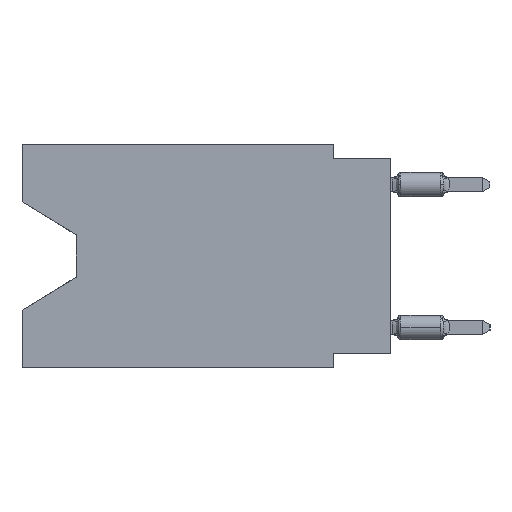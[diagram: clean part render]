
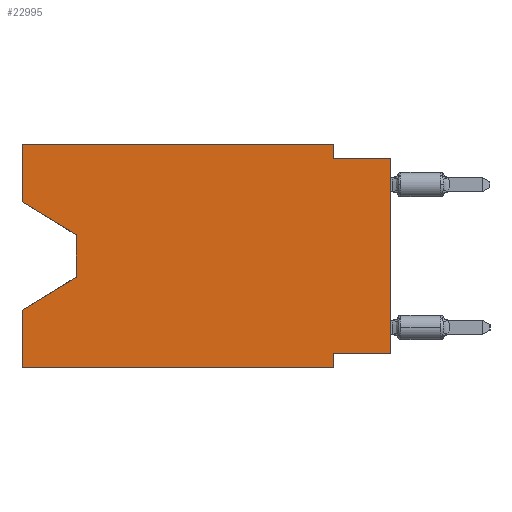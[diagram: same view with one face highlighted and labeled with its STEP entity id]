
A CAD part, left-side view. The second image highlights one B-rep face of the part: STEP entity #22995.
In plain terms, the highlighted planar face has unit normal (-1, 0, 0).
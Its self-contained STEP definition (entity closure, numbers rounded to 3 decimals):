
#367 = CARTESIAN_POINT ( 'NONE',  ( 0., 2.54, -9.906 ) ) ;
#491 = EDGE_LOOP ( 'NONE', ( #17704, #5832, #23189, #4879, #27209, #18446, #586, #12905, #18353, #7124, #14202, #2330 ) ) ;
#516 = VERTEX_POINT ( 'NONE', #23426 ) ;
#586 = ORIENTED_EDGE ( 'NONE', *, *, #18438, .F. ) ;
#728 = EDGE_CURVE ( 'NONE', #2733, #9744, #24272, .T. ) ;
#1650 = LINE ( 'NONE', #8018, #10307 ) ;
#2138 = VERTEX_POINT ( 'NONE', #7632 ) ;
#2330 = ORIENTED_EDGE ( 'NONE', *, *, #15231, .F. ) ;
#2733 = VERTEX_POINT ( 'NONE', #7737 ) ;
#2897 = DIRECTION ( 'NONE',  ( 0., 0., 1. ) ) ;
#3535 = VECTOR ( 'NONE', #8153, 1000. ) ;
#3934 = EDGE_CURVE ( 'NONE', #516, #22753, #12090, .T. ) ;
#4527 = LINE ( 'NONE', #24346, #5271 ) ;
#4879 = ORIENTED_EDGE ( 'NONE', *, *, #18583, .F. ) ;
#5035 = PLANE ( 'NONE',  #27947 ) ;
#5097 = CARTESIAN_POINT ( 'NONE',  ( 0., 16.383, -7.36 ) ) ;
#5271 = VECTOR ( 'NONE', #19856, 1000. ) ;
#5822 = CARTESIAN_POINT ( 'NONE',  ( 0., 16.383, -2.546 ) ) ;
#5832 = ORIENTED_EDGE ( 'NONE', *, *, #3934, .T. ) ;
#6000 = CARTESIAN_POINT ( 'NONE',  ( 0., 13.97, -4.013 ) ) ;
#6475 = CARTESIAN_POINT ( 'NONE',  ( 0., 13.97, -5.893 ) ) ;
#7124 = ORIENTED_EDGE ( 'NONE', *, *, #23572, .F. ) ;
#7632 = CARTESIAN_POINT ( 'NONE',  ( 0., 2.54, -9.271 ) ) ;
#7737 = CARTESIAN_POINT ( 'NONE',  ( 0., 2.54, -0.635 ) ) ;
#8018 = CARTESIAN_POINT ( 'NONE',  ( 0., 16.383, -2.546 ) ) ;
#8153 = DIRECTION ( 'NONE',  ( 0., 0., 1. ) ) ;
#8291 = EDGE_CURVE ( 'NONE', #10574, #18259, #15759, .T. ) ;
#8428 = LINE ( 'NONE', #24194, #14132 ) ;
#8631 = CARTESIAN_POINT ( 'NONE',  ( 0., 16.383, 0. ) ) ;
#9358 = EDGE_CURVE ( 'NONE', #19790, #28056, #4527, .T. ) ;
#9383 = DIRECTION ( 'NONE',  ( 0., -1., 0. ) ) ;
#9526 = VERTEX_POINT ( 'NONE', #12427 ) ;
#9607 = EDGE_CURVE ( 'NONE', #22753, #18701, #10807, .T. ) ;
#9618 = CARTESIAN_POINT ( 'NONE',  ( 0., 0., -9.271 ) ) ;
#9744 = VERTEX_POINT ( 'NONE', #24423 ) ;
#10307 = VECTOR ( 'NONE', #16832, 1000. ) ;
#10445 = VECTOR ( 'NONE', #25067, 1000. ) ;
#10574 = VERTEX_POINT ( 'NONE', #11309 ) ;
#10807 = LINE ( 'NONE', #6475, #17264 ) ;
#11309 = CARTESIAN_POINT ( 'NONE',  ( 0., 16.383, -9.906 ) ) ;
#11474 = VECTOR ( 'NONE', #13114, 1000. ) ;
#11920 = VECTOR ( 'NONE', #12233, 1000. ) ;
#11965 = DIRECTION ( 'NONE',  ( 0., 0., -1. ) ) ;
#12090 = LINE ( 'NONE', #6000, #11920 ) ;
#12186 = CARTESIAN_POINT ( 'NONE',  ( 0., 2.54, -9.906 ) ) ;
#12233 = DIRECTION ( 'NONE',  ( 0., 0., -1. ) ) ;
#12427 = CARTESIAN_POINT ( 'NONE',  ( 0., 0., -9.271 ) ) ;
#12905 = ORIENTED_EDGE ( 'NONE', *, *, #13515, .T. ) ;
#13114 = DIRECTION ( 'NONE',  ( 0., 0., 1. ) ) ;
#13134 = CARTESIAN_POINT ( 'NONE',  ( 0., 0., -0.635 ) ) ;
#13515 = EDGE_CURVE ( 'NONE', #9526, #9744, #27060, .T. ) ;
#13712 = FACE_OUTER_BOUND ( 'NONE', #491, .T. ) ;
#14132 = VECTOR ( 'NONE', #15375, 1000. ) ;
#14202 = ORIENTED_EDGE ( 'NONE', *, *, #9358, .F. ) ;
#14874 = DIRECTION ( 'NONE',  ( 0., 0.855, -0.519 ) ) ;
#15231 = EDGE_CURVE ( 'NONE', #19896, #19790, #15289, .T. ) ;
#15289 = LINE ( 'NONE', #8631, #11474 ) ;
#15375 = DIRECTION ( 'NONE',  ( 0., 0., -1. ) ) ;
#15759 = LINE ( 'NONE', #24723, #25514 ) ;
#16255 = LINE ( 'NONE', #9618, #10445 ) ;
#16832 = DIRECTION ( 'NONE',  ( 0., -0.855, -0.519 ) ) ;
#17120 = EDGE_CURVE ( 'NONE', #2138, #18259, #27808, .T. ) ;
#17264 = VECTOR ( 'NONE', #14874, 1000. ) ;
#17310 = VECTOR ( 'NONE', #21016, 1000. ) ;
#17704 = ORIENTED_EDGE ( 'NONE', *, *, #27121, .T. ) ;
#17840 = CARTESIAN_POINT ( 'NONE',  ( 0., 16.383, 0. ) ) ;
#18248 = VECTOR ( 'NONE', #20603, 1000. ) ;
#18259 = VERTEX_POINT ( 'NONE', #367 ) ;
#18353 = ORIENTED_EDGE ( 'NONE', *, *, #728, .F. ) ;
#18438 = EDGE_CURVE ( 'NONE', #9526, #2138, #16255, .T. ) ;
#18446 = ORIENTED_EDGE ( 'NONE', *, *, #17120, .F. ) ;
#18583 = EDGE_CURVE ( 'NONE', #10574, #18701, #25923, .T. ) ;
#18701 = VERTEX_POINT ( 'NONE', #5097 ) ;
#19405 = CARTESIAN_POINT ( 'NONE',  ( 0., 16.383, 0. ) ) ;
#19790 = VERTEX_POINT ( 'NONE', #17840 ) ;
#19856 = DIRECTION ( 'NONE',  ( 0., -1., 0. ) ) ;
#19896 = VERTEX_POINT ( 'NONE', #5822 ) ;
#20206 = VECTOR ( 'NONE', #2897, 1000. ) ;
#20603 = DIRECTION ( 'NONE',  ( 0., -1., 0. ) ) ;
#20836 = CARTESIAN_POINT ( 'NONE',  ( 0., 0., 0. ) ) ;
#21016 = DIRECTION ( 'NONE',  ( 0., 0., -1. ) ) ;
#21704 = CARTESIAN_POINT ( 'NONE',  ( 0., 13.97, -5.893 ) ) ;
#22753 = VERTEX_POINT ( 'NONE', #21704 ) ;
#22995 = ADVANCED_FACE ( 'NONE', ( #13712 ), #5035, .F. ) ;
#23189 = ORIENTED_EDGE ( 'NONE', *, *, #9607, .T. ) ;
#23426 = CARTESIAN_POINT ( 'NONE',  ( 0., 13.97, -4.013 ) ) ;
#23572 = EDGE_CURVE ( 'NONE', #28056, #2733, #8428, .T. ) ;
#23963 = CARTESIAN_POINT ( 'NONE',  ( 0., 2.54, 0. ) ) ;
#24194 = CARTESIAN_POINT ( 'NONE',  ( 0., 2.54, 0. ) ) ;
#24272 = LINE ( 'NONE', #13134, #18248 ) ;
#24346 = CARTESIAN_POINT ( 'NONE',  ( 0., 16.383, 0. ) ) ;
#24423 = CARTESIAN_POINT ( 'NONE',  ( 0., 0., -0.635 ) ) ;
#24723 = CARTESIAN_POINT ( 'NONE',  ( 0., 16.383, -9.906 ) ) ;
#25067 = DIRECTION ( 'NONE',  ( 0., 1., 0. ) ) ;
#25118 = DIRECTION ( 'NONE',  ( 1., 0., 0. ) ) ;
#25266 = CARTESIAN_POINT ( 'NONE',  ( 0., 16.383, 0. ) ) ;
#25514 = VECTOR ( 'NONE', #9383, 1000. ) ;
#25923 = LINE ( 'NONE', #19405, #3535 ) ;
#27060 = LINE ( 'NONE', #20836, #20206 ) ;
#27121 = EDGE_CURVE ( 'NONE', #19896, #516, #1650, .T. ) ;
#27209 = ORIENTED_EDGE ( 'NONE', *, *, #8291, .T. ) ;
#27808 = LINE ( 'NONE', #12186, #17310 ) ;
#27947 = AXIS2_PLACEMENT_3D ( 'NONE', #25266, #25118, #11965 ) ;
#28056 = VERTEX_POINT ( 'NONE', #23963 ) ;
